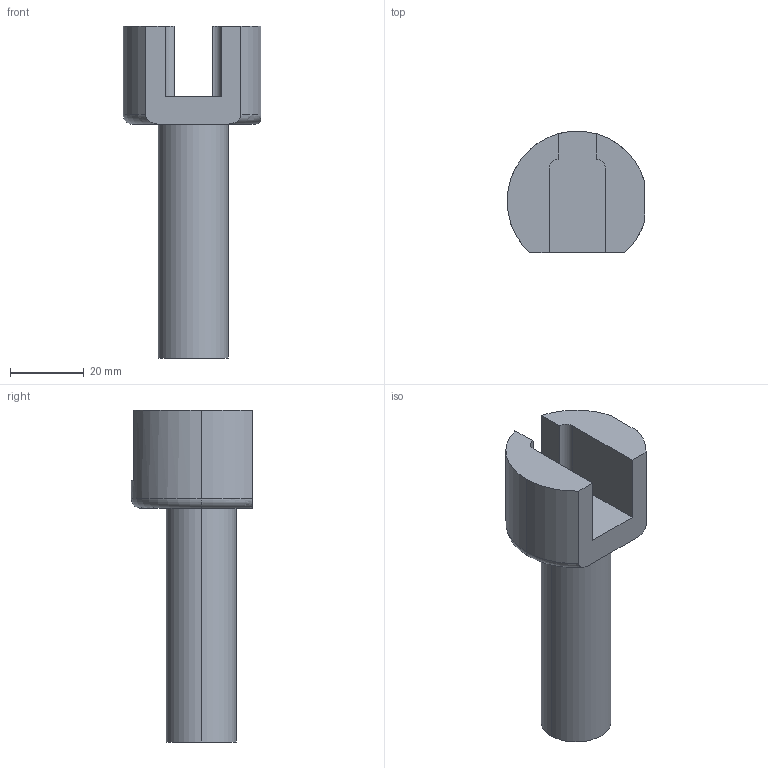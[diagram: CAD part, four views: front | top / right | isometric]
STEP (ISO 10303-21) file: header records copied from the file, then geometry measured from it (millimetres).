
FILE_DESCRIPTION (( 'STEP AP214' ), '1' );
FILE_NAME ('bolt_2.STEP', '2013-11-06T02:13:30', ( '' ), ( '' ), 'SwSTEP 2.0', 'SolidWorks 2013', '' );
FILE_SCHEMA (( 'AUTOMOTIVE_DESIGN' ));
Length unit declared in the file: inch
Products named in the file (1): bolt_2
Bounding box: 37.39 x 33.02 x 90.17 mm (x, y, z)
Volume: 29813.4 mm3; surface area: 12430.1 mm2
Topology: 1 solids, 1 shells, 26 faces, 65 edges, 43 vertices
Faces by surface type: plane 16, cylinder 7, torus 3
Entity records: 884 total; most frequent: CARTESIAN_POINT 205, DIRECTION 136, ORIENTED_EDGE 130, EDGE_CURVE 65, AXIS2_PLACEMENT_3D 48, VERTEX_POINT 43, VECTOR 40, LINE 40
